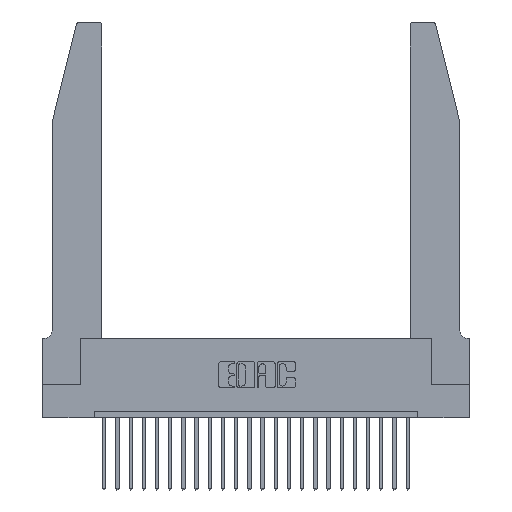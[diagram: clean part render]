
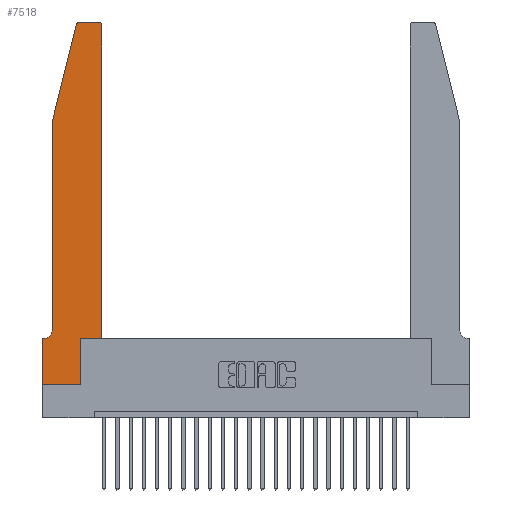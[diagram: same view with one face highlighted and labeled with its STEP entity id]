
A CAD part, top view. The second image highlights one B-rep face of the part: STEP entity #7518.
In plain terms, the highlighted planar face has unit normal (0, 0, 1).
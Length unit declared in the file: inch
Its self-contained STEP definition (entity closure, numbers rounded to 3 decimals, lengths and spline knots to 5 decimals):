
#341 = LINE ( 'NONE', #18807, #15332 ) ;
#394 = LINE ( 'NONE', #11580, #18093 ) ;
#873 = CARTESIAN_POINT ( 'NONE',  ( 0., 0., 0.37 ) ) ;
#948 = EDGE_CURVE ( 'NONE', #16280, #18201, #8963, .T. ) ;
#1169 = EDGE_CURVE ( 'NONE', #5679, #22231, #6516, .T. ) ;
#1209 = CARTESIAN_POINT ( 'NONE',  ( 0.4505, 0.35, 0.37 ) ) ;
#1383 = LINE ( 'NONE', #873, #15122 ) ;
#1513 = LINE ( 'NONE', #19918, #12466 ) ;
#1652 = DIRECTION ( 'NONE',  ( -0.239, -0.971, 0. ) ) ;
#2621 = AXIS2_PLACEMENT_3D ( 'NONE', #14390, #16338, #4676 ) ;
#2635 = CARTESIAN_POINT ( 'NONE',  ( 0., 0.35, 0.37 ) ) ;
#2643 = CARTESIAN_POINT ( 'NONE',  ( 0.0755, 2., 0.37 ) ) ;
#2704 = EDGE_CURVE ( 'NONE', #22261, #2730, #11930, .T. ) ;
#2730 = VERTEX_POINT ( 'NONE', #11368 ) ;
#3408 = ORIENTED_EDGE ( 'NONE', *, *, #24697, .T. ) ;
#3902 = DIRECTION ( 'NONE',  ( 1., 0., 0. ) ) ;
#4024 = ORIENTED_EDGE ( 'NONE', *, *, #8255, .T. ) ;
#4172 = LINE ( 'NONE', #8053, #19130 ) ;
#4676 = DIRECTION ( 'NONE',  ( 1., 0., 0. ) ) ;
#5353 = ORIENTED_EDGE ( 'NONE', *, *, #19748, .T. ) ;
#5679 = VERTEX_POINT ( 'NONE', #18947 ) ;
#6137 = CARTESIAN_POINT ( 'NONE',  ( 0.4505, 2.72, 0.37 ) ) ;
#6516 = LINE ( 'NONE', #21284, #8932 ) ;
#6904 = EDGE_CURVE ( 'NONE', #23110, #5679, #1383, .T. ) ;
#7102 = VECTOR ( 'NONE', #1652, 39.37008 ) ;
#7283 = ORIENTED_EDGE ( 'NONE', *, *, #2704, .T. ) ;
#7518 = ADVANCED_FACE ( 'NONE', ( #22407 ), #24712, .T. ) ;
#8053 = CARTESIAN_POINT ( 'NONE',  ( 0.4505, 0.35, 0.37 ) ) ;
#8255 = EDGE_CURVE ( 'NONE', #17206, #22261, #24227, .T. ) ;
#8394 = DIRECTION ( 'NONE',  ( 0., -1., 0. ) ) ;
#8511 = CARTESIAN_POINT ( 'NONE',  ( 0.4505, 0.35, 0.37 ) ) ;
#8677 = VERTEX_POINT ( 'NONE', #19736 ) ;
#8813 = CARTESIAN_POINT ( 'NONE',  ( 0.0055, 0.35, 0.37 ) ) ;
#8932 = VECTOR ( 'NONE', #9572, 39.37008 ) ;
#8963 = LINE ( 'NONE', #12967, #19974 ) ;
#8968 = ORIENTED_EDGE ( 'NONE', *, *, #13208, .T. ) ;
#9390 = AXIS2_PLACEMENT_3D ( 'NONE', #14646, #14555, #18708 ) ;
#9430 = DIRECTION ( 'NONE',  ( 0., 0., 1. ) ) ;
#9572 = DIRECTION ( 'NONE',  ( 0., 1., 0. ) ) ;
#9778 = EDGE_CURVE ( 'NONE', #22231, #17206, #4172, .T. ) ;
#9849 = EDGE_CURVE ( 'NONE', #14862, #8677, #14564, .T. ) ;
#10066 = ORIENTED_EDGE ( 'NONE', *, *, #1169, .T. ) ;
#10112 = CARTESIAN_POINT ( 'NONE',  ( 0.0755, 0.42, 0.37 ) ) ;
#10217 = DIRECTION ( 'NONE',  ( 1., 0., 0. ) ) ;
#10276 = DIRECTION ( 'NONE',  ( 0., 0., -1. ) ) ;
#10773 = LINE ( 'NONE', #24118, #7102 ) ;
#10803 = CIRCLE ( 'NONE', #11491, 0.07 ) ;
#10876 = DIRECTION ( 'NONE',  ( -1., 0., 0. ) ) ;
#11142 = ORIENTED_EDGE ( 'NONE', *, *, #24397, .T. ) ;
#11368 = CARTESIAN_POINT ( 'NONE',  ( 0.4205, 2.75, 0.37 ) ) ;
#11491 = AXIS2_PLACEMENT_3D ( 'NONE', #16027, #10276, #12362 ) ;
#11580 = CARTESIAN_POINT ( 'NONE',  ( 0., 0., 0.37 ) ) ;
#11930 = CIRCLE ( 'NONE', #2621, 0.03 ) ;
#12077 = EDGE_CURVE ( 'NONE', #8677, #17036, #10773, .T. ) ;
#12362 = DIRECTION ( 'NONE',  ( -1., 0., 0. ) ) ;
#12466 = VECTOR ( 'NONE', #8394, 39.37008 ) ;
#12967 = CARTESIAN_POINT ( 'NONE',  ( 0.0755, 0.35, 0.37 ) ) ;
#13208 = EDGE_CURVE ( 'NONE', #2730, #14862, #341, .T. ) ;
#13443 = EDGE_LOOP ( 'NONE', ( #8968, #14735, #23417, #5353, #11142, #21066, #3408, #15434, #10066, #24659, #4024, #7283 ) ) ;
#13869 = VECTOR ( 'NONE', #22624, 39.37008 ) ;
#14261 = CARTESIAN_POINT ( 'NONE',  ( 0.2865, 0.35, 0.37 ) ) ;
#14390 = CARTESIAN_POINT ( 'NONE',  ( 0.4205, 2.72, 0.37 ) ) ;
#14555 = DIRECTION ( 'NONE',  ( 0., 0., 1. ) ) ;
#14564 = CIRCLE ( 'NONE', #9390, 0.03 ) ;
#14646 = CARTESIAN_POINT ( 'NONE',  ( 0.284, 2.72, 0.37 ) ) ;
#14735 = ORIENTED_EDGE ( 'NONE', *, *, #9849, .T. ) ;
#14862 = VERTEX_POINT ( 'NONE', #23470 ) ;
#15122 = VECTOR ( 'NONE', #10217, 39.37008 ) ;
#15332 = VECTOR ( 'NONE', #10876, 39.37008 ) ;
#15434 = ORIENTED_EDGE ( 'NONE', *, *, #6904, .T. ) ;
#16027 = CARTESIAN_POINT ( 'NONE',  ( 0.0055, 0.42, 0.37 ) ) ;
#16280 = VERTEX_POINT ( 'NONE', #8813 ) ;
#16338 = DIRECTION ( 'NONE',  ( 0., 0., 1. ) ) ;
#16385 = VERTEX_POINT ( 'NONE', #10112 ) ;
#16582 = AXIS2_PLACEMENT_3D ( 'NONE', #2635, #9430, #25038 ) ;
#17036 = VERTEX_POINT ( 'NONE', #2643 ) ;
#17048 = DIRECTION ( 'NONE',  ( -1., 0., 0. ) ) ;
#17206 = VERTEX_POINT ( 'NONE', #8511 ) ;
#18093 = VECTOR ( 'NONE', #20710, 39.37008 ) ;
#18201 = VERTEX_POINT ( 'NONE', #22557 ) ;
#18708 = DIRECTION ( 'NONE',  ( 1., 0., 0. ) ) ;
#18807 = CARTESIAN_POINT ( 'NONE',  ( 0.2605, 2.75, 0.37 ) ) ;
#18947 = CARTESIAN_POINT ( 'NONE',  ( 0.2865, 0., 0.37 ) ) ;
#19130 = VECTOR ( 'NONE', #3902, 39.37008 ) ;
#19736 = CARTESIAN_POINT ( 'NONE',  ( 0.25487, 2.72718, 0.37 ) ) ;
#19748 = EDGE_CURVE ( 'NONE', #17036, #16385, #1513, .T. ) ;
#19918 = CARTESIAN_POINT ( 'NONE',  ( 0.0755, 2., 0.37 ) ) ;
#19974 = VECTOR ( 'NONE', #17048, 39.37008 ) ;
#20710 = DIRECTION ( 'NONE',  ( 0., -1., 0. ) ) ;
#21066 = ORIENTED_EDGE ( 'NONE', *, *, #948, .T. ) ;
#21284 = CARTESIAN_POINT ( 'NONE',  ( 0.2865, 0.35, 0.37 ) ) ;
#22231 = VERTEX_POINT ( 'NONE', #14261 ) ;
#22261 = VERTEX_POINT ( 'NONE', #6137 ) ;
#22309 = CARTESIAN_POINT ( 'NONE',  ( 0., 0., 0.37 ) ) ;
#22407 = FACE_OUTER_BOUND ( 'NONE', #13443, .T. ) ;
#22557 = CARTESIAN_POINT ( 'NONE',  ( 0., 0.35, 0.37 ) ) ;
#22624 = DIRECTION ( 'NONE',  ( 0., 1., 0. ) ) ;
#23110 = VERTEX_POINT ( 'NONE', #22309 ) ;
#23417 = ORIENTED_EDGE ( 'NONE', *, *, #12077, .T. ) ;
#23470 = CARTESIAN_POINT ( 'NONE',  ( 0.284, 2.75, 0.37 ) ) ;
#24118 = CARTESIAN_POINT ( 'NONE',  ( 0.0755, 2., 0.37 ) ) ;
#24227 = LINE ( 'NONE', #1209, #13869 ) ;
#24397 = EDGE_CURVE ( 'NONE', #16385, #16280, #10803, .T. ) ;
#24659 = ORIENTED_EDGE ( 'NONE', *, *, #9778, .T. ) ;
#24697 = EDGE_CURVE ( 'NONE', #18201, #23110, #394, .T. ) ;
#24712 = PLANE ( 'NONE',  #16582 ) ;
#25038 = DIRECTION ( 'NONE',  ( 1., 0., 0. ) ) ;
